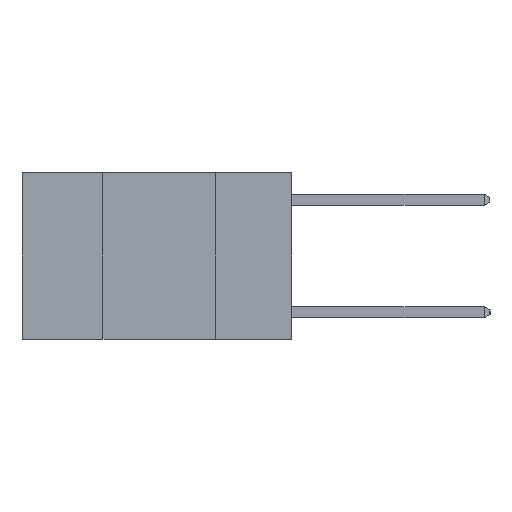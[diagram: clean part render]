
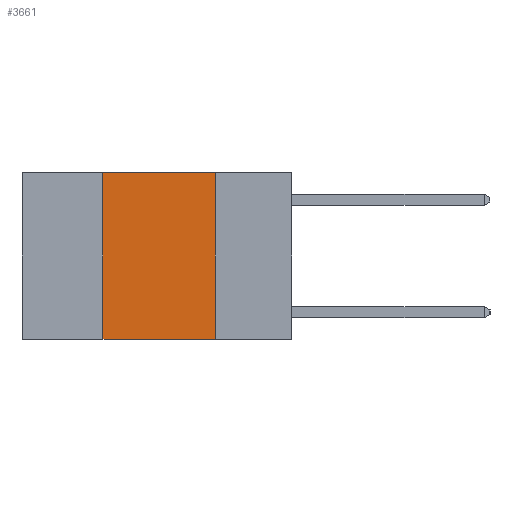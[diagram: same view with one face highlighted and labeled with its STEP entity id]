
A CAD part, left-side view. The second image highlights one B-rep face of the part: STEP entity #3661.
In plain terms, the highlighted planar face has unit normal (-1, 0, 0).
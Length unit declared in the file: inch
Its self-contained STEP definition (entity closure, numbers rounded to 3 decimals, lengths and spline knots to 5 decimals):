
#144 = DIRECTION ( 'NONE',  ( 1., 0., 0. ) ) ;
#604 = LINE ( 'NONE', #8624, #2236 ) ;
#1747 = AXIS2_PLACEMENT_3D ( 'NONE', #7450, #144, #3626 ) ;
#2001 = ORIENTED_EDGE ( 'NONE', *, *, #3363, .T. ) ;
#2098 = DIRECTION ( 'NONE',  ( 0., 0., 1. ) ) ;
#2170 = FACE_OUTER_BOUND ( 'NONE', #7407, .T. ) ;
#2236 = VECTOR ( 'NONE', #2616, 39.37008 ) ;
#2358 = VERTEX_POINT ( 'NONE', #7482 ) ;
#2599 = DIRECTION ( 'NONE',  ( 0., -1., 0. ) ) ;
#2616 = DIRECTION ( 'NONE',  ( 0., -1., 0. ) ) ;
#2965 = ORIENTED_EDGE ( 'NONE', *, *, #5648, .F. ) ;
#3326 = CARTESIAN_POINT ( 'NONE',  ( 0., 0.17, 0. ) ) ;
#3363 = EDGE_CURVE ( 'NONE', #4947, #3900, #6007, .T. ) ;
#3577 = VECTOR ( 'NONE', #2098, 39.37008 ) ;
#3626 = DIRECTION ( 'NONE',  ( 0., 0., -1. ) ) ;
#3661 = ADVANCED_FACE ( 'NONE', ( #2170 ), #6176, .F. ) ;
#3718 = EDGE_CURVE ( 'NONE', #6729, #3900, #8663, .T. ) ;
#3900 = VERTEX_POINT ( 'NONE', #4124 ) ;
#3991 = ORIENTED_EDGE ( 'NONE', *, *, #6013, .F. ) ;
#4124 = CARTESIAN_POINT ( 'NONE',  ( 0., 0.17, -0.37 ) ) ;
#4395 = DIRECTION ( 'NONE',  ( 0., 0., -1. ) ) ;
#4424 = VECTOR ( 'NONE', #2599, 39.37008 ) ;
#4947 = VERTEX_POINT ( 'NONE', #8080 ) ;
#5234 = ORIENTED_EDGE ( 'NONE', *, *, #3718, .F. ) ;
#5322 = LINE ( 'NONE', #5378, #3577 ) ;
#5378 = CARTESIAN_POINT ( 'NONE',  ( 0., 0.42, 0. ) ) ;
#5462 = CARTESIAN_POINT ( 'NONE',  ( 0., 0.17, 0. ) ) ;
#5648 = EDGE_CURVE ( 'NONE', #4947, #2358, #5322, .T. ) ;
#6007 = LINE ( 'NONE', #6045, #4424 ) ;
#6013 = EDGE_CURVE ( 'NONE', #2358, #6729, #604, .T. ) ;
#6045 = CARTESIAN_POINT ( 'NONE',  ( 0., 0.6, -0.37 ) ) ;
#6176 = PLANE ( 'NONE',  #1747 ) ;
#6729 = VERTEX_POINT ( 'NONE', #3326 ) ;
#6833 = VECTOR ( 'NONE', #4395, 39.37008 ) ;
#7407 = EDGE_LOOP ( 'NONE', ( #5234, #3991, #2965, #2001 ) ) ;
#7450 = CARTESIAN_POINT ( 'NONE',  ( 0., 0.6, 0. ) ) ;
#7482 = CARTESIAN_POINT ( 'NONE',  ( 0., 0.42, 0. ) ) ;
#8080 = CARTESIAN_POINT ( 'NONE',  ( 0., 0.42, -0.37 ) ) ;
#8624 = CARTESIAN_POINT ( 'NONE',  ( 0., 0.6, 0. ) ) ;
#8663 = LINE ( 'NONE', #5462, #6833 ) ;
